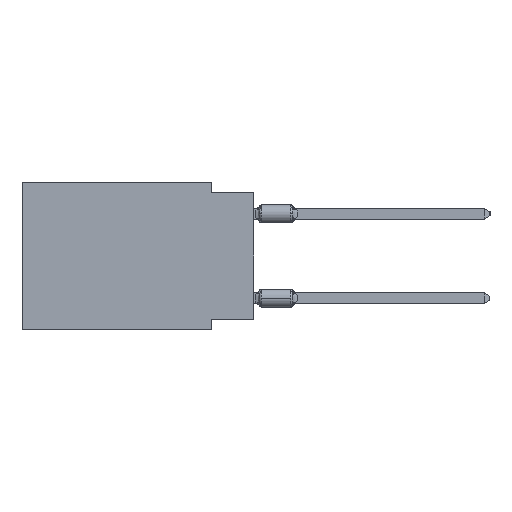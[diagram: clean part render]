
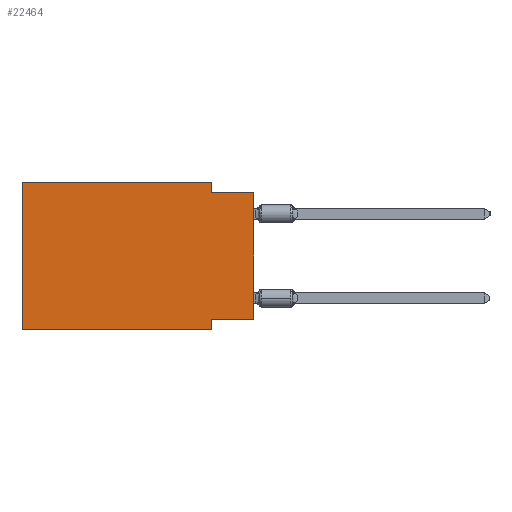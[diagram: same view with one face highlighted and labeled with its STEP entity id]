
A CAD part, left-side view. The second image highlights one B-rep face of the part: STEP entity #22464.
In plain terms, the highlighted planar face has unit normal (-1, 0, 0).
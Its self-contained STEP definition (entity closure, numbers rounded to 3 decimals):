
#44 = EDGE_CURVE ( 'NONE', #563, #721, #9251, .T. ) ;
#221 = VECTOR ( 'NONE', #2750, 1000. ) ;
#563 = VERTEX_POINT ( 'NONE', #34229 ) ;
#721 = VERTEX_POINT ( 'NONE', #8659 ) ;
#732 = VECTOR ( 'NONE', #29599, 1000. ) ;
#1321 = VERTEX_POINT ( 'NONE', #19842 ) ;
#1716 = AXIS2_PLACEMENT_3D ( 'NONE', #23611, #11265, #30332 ) ;
#2193 = CARTESIAN_POINT ( 'NONE',  ( 0., 0., -0.635 ) ) ;
#2651 = EDGE_CURVE ( 'NONE', #1321, #4846, #3597, .T. ) ;
#2731 = VERTEX_POINT ( 'NONE', #20480 ) ;
#2750 = DIRECTION ( 'NONE',  ( 0., -1., 0. ) ) ;
#3597 = LINE ( 'NONE', #16809, #15328 ) ;
#3912 = CARTESIAN_POINT ( 'NONE',  ( 0., 13.97, 0. ) ) ;
#4846 = VERTEX_POINT ( 'NONE', #11623 ) ;
#6414 = CARTESIAN_POINT ( 'NONE',  ( 0., 2.54, 0. ) ) ;
#7228 = EDGE_CURVE ( 'NONE', #2731, #7519, #20560, .T. ) ;
#7386 = EDGE_CURVE ( 'NONE', #39366, #28800, #28372, .T. ) ;
#7519 = VERTEX_POINT ( 'NONE', #22295 ) ;
#8012 = CARTESIAN_POINT ( 'NONE',  ( 0., 13.97, 0. ) ) ;
#8659 = CARTESIAN_POINT ( 'NONE',  ( 0., 2.54, -0.635 ) ) ;
#9251 = LINE ( 'NONE', #6414, #732 ) ;
#9885 = ORIENTED_EDGE ( 'NONE', *, *, #21316, .T. ) ;
#10393 = DIRECTION ( 'NONE',  ( 0., 0., -1. ) ) ;
#11265 = DIRECTION ( 'NONE',  ( 1., 0., 0. ) ) ;
#11623 = CARTESIAN_POINT ( 'NONE',  ( 0., 0., -0.635 ) ) ;
#11815 = CARTESIAN_POINT ( 'NONE',  ( 0., 13.97, -8.89 ) ) ;
#12375 = DIRECTION ( 'NONE',  ( 0., -1., 0. ) ) ;
#13885 = ORIENTED_EDGE ( 'NONE', *, *, #44, .F. ) ;
#15313 = CARTESIAN_POINT ( 'NONE',  ( 0., 13.97, -8.89 ) ) ;
#15328 = VECTOR ( 'NONE', #30040, 1000. ) ;
#15970 = EDGE_CURVE ( 'NONE', #1321, #2731, #42072, .T. ) ;
#16059 = LINE ( 'NONE', #21909, #23661 ) ;
#16319 = ORIENTED_EDGE ( 'NONE', *, *, #15970, .F. ) ;
#16419 = LINE ( 'NONE', #2193, #32694 ) ;
#16809 = CARTESIAN_POINT ( 'NONE',  ( 0., 0., 0. ) ) ;
#17315 = FACE_OUTER_BOUND ( 'NONE', #27279, .T. ) ;
#17721 = EDGE_CURVE ( 'NONE', #721, #4846, #16419, .T. ) ;
#19144 = VECTOR ( 'NONE', #10393, 1000. ) ;
#19842 = CARTESIAN_POINT ( 'NONE',  ( 0., 0., -8.255 ) ) ;
#20480 = CARTESIAN_POINT ( 'NONE',  ( 0., 2.54, -8.255 ) ) ;
#20560 = LINE ( 'NONE', #23395, #19144 ) ;
#21316 = EDGE_CURVE ( 'NONE', #39366, #7519, #38950, .T. ) ;
#21722 = VECTOR ( 'NONE', #22325, 1000. ) ;
#21737 = ORIENTED_EDGE ( 'NONE', *, *, #41361, .F. ) ;
#21909 = CARTESIAN_POINT ( 'NONE',  ( 0., 13.97, 0. ) ) ;
#22295 = CARTESIAN_POINT ( 'NONE',  ( 0., 2.54, -8.89 ) ) ;
#22325 = DIRECTION ( 'NONE',  ( 0., 1., 0. ) ) ;
#22464 = ADVANCED_FACE ( 'NONE', ( #17315 ), #40958, .F. ) ;
#22560 = DIRECTION ( 'NONE',  ( 0., -1., 0. ) ) ;
#23395 = CARTESIAN_POINT ( 'NONE',  ( 0., 2.54, -8.89 ) ) ;
#23611 = CARTESIAN_POINT ( 'NONE',  ( 0., 13.97, 0. ) ) ;
#23661 = VECTOR ( 'NONE', #22560, 1000. ) ;
#24889 = DIRECTION ( 'NONE',  ( 0., 0., 1. ) ) ;
#25362 = VECTOR ( 'NONE', #24889, 1000. ) ;
#27279 = EDGE_LOOP ( 'NONE', ( #35299, #30520, #13885, #21737, #42031, #9885, #31127, #16319 ) ) ;
#28372 = LINE ( 'NONE', #8012, #25362 ) ;
#28403 = CARTESIAN_POINT ( 'NONE',  ( 0., 0., -8.255 ) ) ;
#28800 = VERTEX_POINT ( 'NONE', #3912 ) ;
#29599 = DIRECTION ( 'NONE',  ( 0., 0., -1. ) ) ;
#30040 = DIRECTION ( 'NONE',  ( 0., 0., 1. ) ) ;
#30332 = DIRECTION ( 'NONE',  ( 0., 0., -1. ) ) ;
#30520 = ORIENTED_EDGE ( 'NONE', *, *, #17721, .F. ) ;
#31127 = ORIENTED_EDGE ( 'NONE', *, *, #7228, .F. ) ;
#32694 = VECTOR ( 'NONE', #12375, 1000. ) ;
#34229 = CARTESIAN_POINT ( 'NONE',  ( 0., 2.54, 0. ) ) ;
#35299 = ORIENTED_EDGE ( 'NONE', *, *, #2651, .T. ) ;
#38950 = LINE ( 'NONE', #15313, #221 ) ;
#39366 = VERTEX_POINT ( 'NONE', #11815 ) ;
#40958 = PLANE ( 'NONE',  #1716 ) ;
#41361 = EDGE_CURVE ( 'NONE', #28800, #563, #16059, .T. ) ;
#42031 = ORIENTED_EDGE ( 'NONE', *, *, #7386, .F. ) ;
#42072 = LINE ( 'NONE', #28403, #21722 ) ;
